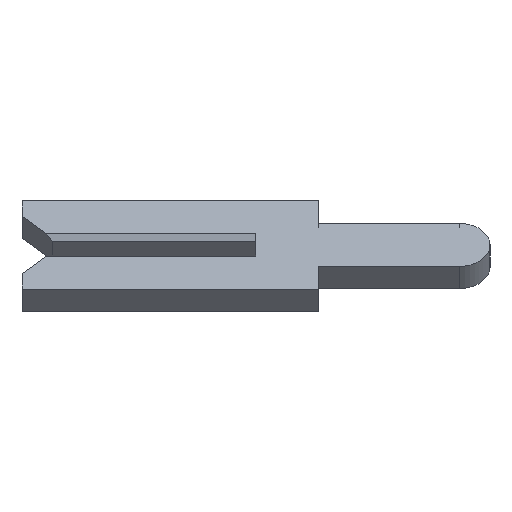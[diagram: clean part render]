
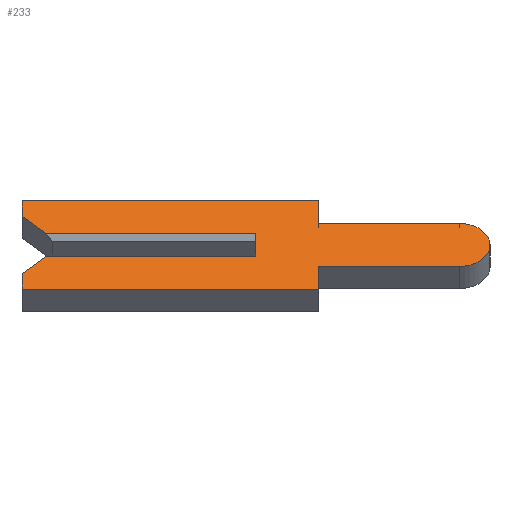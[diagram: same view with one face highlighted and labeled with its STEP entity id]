
A CAD part, left-side view. The second image highlights one B-rep face of the part: STEP entity #233.
In plain terms, the highlighted face is planar.
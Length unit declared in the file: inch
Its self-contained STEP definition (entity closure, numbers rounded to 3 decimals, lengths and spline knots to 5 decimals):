
#12 = CARTESIAN_POINT ( 'NONE',  ( -0.01, 0., 0.0065 ) ) ;
#28 = CARTESIAN_POINT ( 'NONE',  ( -0.01, -0.04, 0.04 ) ) ;
#42 = VECTOR ( 'NONE', #936, 39.37008 ) ;
#43 = EDGE_CURVE ( 'NONE', #620, #298, #590, .T. ) ;
#47 = CARTESIAN_POINT ( 'NONE',  ( -0.01, -0.1305, 0. ) ) ;
#64 = LINE ( 'NONE', #292, #424 ) ;
#68 = ORIENTED_EDGE ( 'NONE', *, *, #297, .T. ) ;
#75 = VERTEX_POINT ( 'NONE', #441 ) ;
#80 = ORIENTED_EDGE ( 'NONE', *, *, #105, .F. ) ;
#99 = CARTESIAN_POINT ( 'NONE',  ( -0.01, 0.15, -0.026 ) ) ;
#105 = EDGE_CURVE ( 'NONE', #913, #201, #780, .T. ) ;
#109 = ORIENTED_EDGE ( 'NONE', *, *, #560, .F. ) ;
#114 = VECTOR ( 'NONE', #726, 39.37008 ) ;
#142 = VERTEX_POINT ( 'NONE', #845 ) ;
#155 = AXIS2_PLACEMENT_3D ( 'NONE', #47, #612, #1015 ) ;
#159 = CARTESIAN_POINT ( 'NONE',  ( -0.01, -0.1305, -0.01 ) ) ;
#165 = EDGE_CURVE ( 'NONE', #75, #632, #306, .T. ) ;
#173 = LINE ( 'NONE', #959, #196 ) ;
#186 = VECTOR ( 'NONE', #305, 39.37008 ) ;
#190 = CARTESIAN_POINT ( 'NONE',  ( -0.01, 0.15, -0.04 ) ) ;
#196 = VECTOR ( 'NONE', #479, 39.37008 ) ;
#201 = VERTEX_POINT ( 'NONE', #626 ) ;
#222 = CARTESIAN_POINT ( 'NONE',  ( -0.01, 0.15, -0.026 ) ) ;
#233 = ADVANCED_FACE ( 'NONE', ( #445 ), #775, .F. ) ;
#240 = CARTESIAN_POINT ( 'NONE',  ( -0.01, -0.04, -0.0195 ) ) ;
#255 = LINE ( 'NONE', #159, #186 ) ;
#259 = EDGE_CURVE ( 'NONE', #964, #974, #538, .T. ) ;
#268 = ORIENTED_EDGE ( 'NONE', *, *, #303, .F. ) ;
#270 = CARTESIAN_POINT ( 'NONE',  ( -0.01, -0.04, -0.04 ) ) ;
#281 = DIRECTION ( 'NONE',  ( 0., 0., 1. ) ) ;
#285 = VECTOR ( 'NONE', #817, 39.37008 ) ;
#291 = VECTOR ( 'NONE', #374, 39.37008 ) ;
#292 = CARTESIAN_POINT ( 'NONE',  ( -0.01, 0.15, 0.04 ) ) ;
#297 = EDGE_CURVE ( 'NONE', #345, #772, #592, .T. ) ;
#298 = VERTEX_POINT ( 'NONE', #539 ) ;
#303 = EDGE_CURVE ( 'NONE', #658, #75, #64, .T. ) ;
#305 = DIRECTION ( 'NONE',  ( 0., -1., 0. ) ) ;
#306 = LINE ( 'NONE', #28, #933 ) ;
#311 = CARTESIAN_POINT ( 'NONE',  ( -0.01, 0.15, 0.026 ) ) ;
#321 = VECTOR ( 'NONE', #362, 39.37008 ) ;
#326 = EDGE_CURVE ( 'NONE', #345, #452, #368, .T. ) ;
#344 = ORIENTED_EDGE ( 'NONE', *, *, #934, .F. ) ;
#345 = VERTEX_POINT ( 'NONE', #1021 ) ;
#359 = DIRECTION ( 'NONE',  ( 1., 0., 0. ) ) ;
#362 = DIRECTION ( 'NONE',  ( 0., 0.707, 0.707 ) ) ;
#368 = LINE ( 'NONE', #857, #321 ) ;
#374 = DIRECTION ( 'NONE',  ( 0., -1., 0. ) ) ;
#379 = ORIENTED_EDGE ( 'NONE', *, *, #468, .F. ) ;
#405 = EDGE_CURVE ( 'NONE', #142, #953, #255, .T. ) ;
#406 = VECTOR ( 'NONE', #555, 39.37008 ) ;
#418 = DIRECTION ( 'NONE',  ( 0., 0., 1. ) ) ;
#424 = VECTOR ( 'NONE', #869, 39.37008 ) ;
#441 = CARTESIAN_POINT ( 'NONE',  ( -0.01, -0.04, 0.04 ) ) ;
#443 = DIRECTION ( 'NONE',  ( 0., 0., -1. ) ) ;
#445 = FACE_OUTER_BOUND ( 'NONE', #727, .T. ) ;
#449 = CARTESIAN_POINT ( 'NONE',  ( -0.01, 0.15, 0.01 ) ) ;
#452 = VERTEX_POINT ( 'NONE', #311 ) ;
#468 = EDGE_CURVE ( 'NONE', #452, #658, #636, .T. ) ;
#471 = VECTOR ( 'NONE', #810, 39.37008 ) ;
#479 = DIRECTION ( 'NONE',  ( 0., -1., 0. ) ) ;
#488 = ORIENTED_EDGE ( 'NONE', *, *, #405, .F. ) ;
#501 = EDGE_CURVE ( 'NONE', #632, #913, #173, .T. ) ;
#504 = LINE ( 'NONE', #570, #285 ) ;
#521 = EDGE_CURVE ( 'NONE', #298, #964, #695, .T. ) ;
#538 = LINE ( 'NONE', #222, #753 ) ;
#539 = CARTESIAN_POINT ( 'NONE',  ( -0.01, -0.04, -0.04 ) ) ;
#555 = DIRECTION ( 'NONE',  ( 0., 1., 0. ) ) ;
#560 = EDGE_CURVE ( 'NONE', #201, #620, #978, .T. ) ;
#570 = CARTESIAN_POINT ( 'NONE',  ( -0.01, 0.1305, -0.0065 ) ) ;
#571 = AXIS2_PLACEMENT_3D ( 'NONE', #997, #359, #443 ) ;
#590 = LINE ( 'NONE', #270, #42 ) ;
#592 = LINE ( 'NONE', #449, #291 ) ;
#612 = DIRECTION ( 'NONE',  ( 1., 0., 0. ) ) ;
#620 = VERTEX_POINT ( 'NONE', #240 ) ;
#626 = CARTESIAN_POINT ( 'NONE',  ( -0.01, -0.1305, -0.0195 ) ) ;
#632 = VERTEX_POINT ( 'NONE', #821 ) ;
#636 = LINE ( 'NONE', #643, #114 ) ;
#643 = CARTESIAN_POINT ( 'NONE',  ( -0.01, 0.15, 0.026 ) ) ;
#658 = VERTEX_POINT ( 'NONE', #907 ) ;
#663 = CARTESIAN_POINT ( 'NONE',  ( -0.01, 0., 0.01 ) ) ;
#665 = ORIENTED_EDGE ( 'NONE', *, *, #259, .F. ) ;
#693 = EDGE_CURVE ( 'NONE', #974, #142, #504, .T. ) ;
#695 = LINE ( 'NONE', #876, #406 ) ;
#726 = DIRECTION ( 'NONE',  ( 0., 0., 1. ) ) ;
#727 = EDGE_LOOP ( 'NONE', ( #68, #344, #488, #852, #665, #914, #842, #109, #80, #814, #827, #268, #379, #740 ) ) ;
#740 = ORIENTED_EDGE ( 'NONE', *, *, #326, .F. ) ;
#745 = CARTESIAN_POINT ( 'NONE',  ( -0.01, -0.1305, 0.0195 ) ) ;
#753 = VECTOR ( 'NONE', #281, 39.37008 ) ;
#772 = VERTEX_POINT ( 'NONE', #663 ) ;
#775 = PLANE ( 'NONE',  #155 ) ;
#780 = CIRCLE ( 'NONE', #571, 0.0195 ) ;
#810 = DIRECTION ( 'NONE',  ( 0., 1., 0. ) ) ;
#814 = ORIENTED_EDGE ( 'NONE', *, *, #501, .F. ) ;
#817 = DIRECTION ( 'NONE',  ( 0., -0.707, 0.707 ) ) ;
#821 = CARTESIAN_POINT ( 'NONE',  ( -0.01, -0.04, 0.0195 ) ) ;
#827 = ORIENTED_EDGE ( 'NONE', *, *, #165, .F. ) ;
#842 = ORIENTED_EDGE ( 'NONE', *, *, #43, .F. ) ;
#844 = CARTESIAN_POINT ( 'NONE',  ( -0.01, 0., -0.01 ) ) ;
#845 = CARTESIAN_POINT ( 'NONE',  ( -0.01, 0.134, -0.01 ) ) ;
#852 = ORIENTED_EDGE ( 'NONE', *, *, #693, .F. ) ;
#857 = CARTESIAN_POINT ( 'NONE',  ( -0.01, 0.1305, 0.0065 ) ) ;
#869 = DIRECTION ( 'NONE',  ( 0., -1., 0. ) ) ;
#876 = CARTESIAN_POINT ( 'NONE',  ( -0.01, 0.15, -0.04 ) ) ;
#907 = CARTESIAN_POINT ( 'NONE',  ( -0.01, 0.15, 0.04 ) ) ;
#913 = VERTEX_POINT ( 'NONE', #745 ) ;
#914 = ORIENTED_EDGE ( 'NONE', *, *, #521, .F. ) ;
#933 = VECTOR ( 'NONE', #943, 39.37008 ) ;
#934 = EDGE_CURVE ( 'NONE', #953, #772, #1044, .T. ) ;
#936 = DIRECTION ( 'NONE',  ( 0., 0., -1. ) ) ;
#943 = DIRECTION ( 'NONE',  ( 0., 0., -1. ) ) ;
#953 = VERTEX_POINT ( 'NONE', #844 ) ;
#959 = CARTESIAN_POINT ( 'NONE',  ( -0.01, -0.04, 0.0195 ) ) ;
#964 = VERTEX_POINT ( 'NONE', #190 ) ;
#966 = CARTESIAN_POINT ( 'NONE',  ( -0.01, -0.04, -0.0195 ) ) ;
#974 = VERTEX_POINT ( 'NONE', #99 ) ;
#978 = LINE ( 'NONE', #966, #471 ) ;
#985 = VECTOR ( 'NONE', #418, 39.37008 ) ;
#997 = CARTESIAN_POINT ( 'NONE',  ( -0.01, -0.1305, 0. ) ) ;
#1015 = DIRECTION ( 'NONE',  ( 0., 0., -1. ) ) ;
#1021 = CARTESIAN_POINT ( 'NONE',  ( -0.01, 0.134, 0.01 ) ) ;
#1044 = LINE ( 'NONE', #12, #985 ) ;
